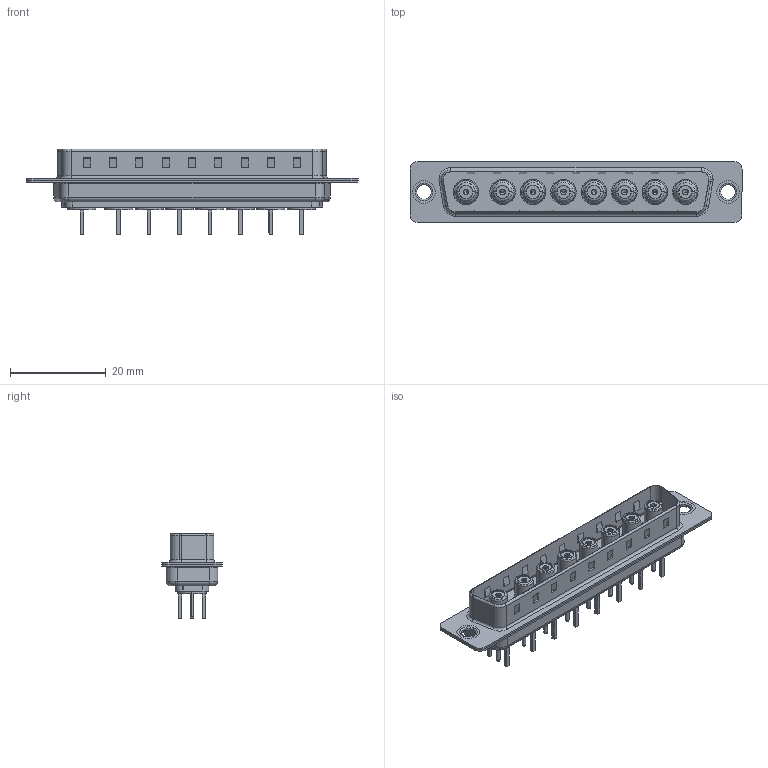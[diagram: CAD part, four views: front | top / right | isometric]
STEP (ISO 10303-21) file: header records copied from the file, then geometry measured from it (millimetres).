
FILE_DESCRIPTION (( 'STEP AP203' ), '1' );
FILE_NAME ('627-8W8-624-5N1.STEP', '2019-05-28T05:52:09', ( '' ), ( '' ), 'SwSTEP 2.0', 'SolidWorks 2016', '' );
FILE_SCHEMA (( 'CONFIG_CONTROL_DESIGN' ));
Length unit declared in the file: millimetre
Products named in the file (11): 627Combo Shell Rear_37 Contacts; Co-Ax Jack Assy_S; Insulator Socket 2; Socket_Str; 627Combo Thru Hole Rivet; 627Combo Housing_8W8; Insulator Socket; Locking Collar; 627Combo Shell Front_37 Contacts; Co-Ax Jack_Straight PC Tail; 627-8W8-624-5N1
Assembly tree (18 placements, depth 3):
  627-8W8-624-5N1
    627Combo Housing_8W8
    627Combo Shell Rear_37 Contacts
    627Combo Shell Front_37 Contacts
    627Combo Thru Hole Rivet  x2
    Co-Ax Jack Assy_S  x8
      Co-Ax Jack_Straight PC Tail
      Insulator Socket
      Insulator Socket 2
      Locking Collar
      Socket_Str
Bounding box: 69.3 x 12.6 x 17.9 mm (x, y, z)
Volume: 3874.2 mm3; surface area: 12322.1 mm2
Topology: 45 solids, 45 shells, 1274 faces, 2967 edges, 1858 vertices
Faces by surface type: plane 579, cylinder 501, torus 90, cone 72, bspline 16, sphere 16
Entity records: 16770 total; most frequent: DIRECTION 2776, CARTESIAN_POINT 2742, ORIENTED_EDGE 2524, EDGE_CURVE 1262, AXIS2_PLACEMENT_3D 1009, VERTEX_POINT 798, LINE 758, VECTOR 758
